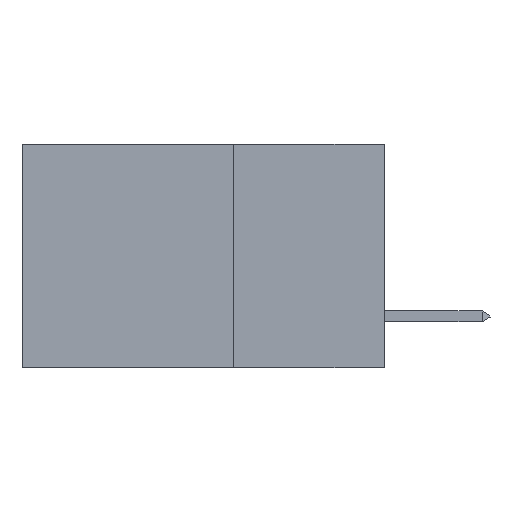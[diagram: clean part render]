
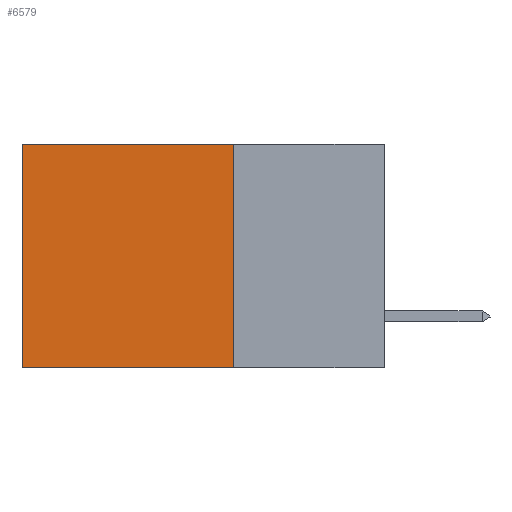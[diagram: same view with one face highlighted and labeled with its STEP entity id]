
A CAD part, left-side view. The second image highlights one B-rep face of the part: STEP entity #6579.
In plain terms, the highlighted planar face has unit normal (-1, 0, 0).
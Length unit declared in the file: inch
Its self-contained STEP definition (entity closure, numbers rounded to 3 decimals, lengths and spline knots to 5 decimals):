
#122 = EDGE_CURVE ( 'NONE', #7248, #6444, #5479, .T. ) ;
#138 = LINE ( 'NONE', #6933, #7232 ) ;
#564 = CARTESIAN_POINT ( 'NONE',  ( 0.2875, 0.25, -0.37 ) ) ;
#593 = CARTESIAN_POINT ( 'NONE',  ( 0.2875, 0.25, -0.37 ) ) ;
#656 = CARTESIAN_POINT ( 'NONE',  ( 0.2875, 0.25, 0. ) ) ;
#776 = ORIENTED_EDGE ( 'NONE', *, *, #122, .T. ) ;
#1270 = ORIENTED_EDGE ( 'NONE', *, *, #9127, .F. ) ;
#1490 = LINE ( 'NONE', #2116, #5525 ) ;
#1652 = CARTESIAN_POINT ( 'NONE',  ( 0.2875, 0.25, 0. ) ) ;
#2116 = CARTESIAN_POINT ( 'NONE',  ( 0.2875, 0.25, 0. ) ) ;
#2440 = VERTEX_POINT ( 'NONE', #564 ) ;
#2858 = DIRECTION ( 'NONE',  ( 0., 0., -1. ) ) ;
#2945 = EDGE_LOOP ( 'NONE', ( #3416, #3709, #1270, #776 ) ) ;
#3397 = VECTOR ( 'NONE', #7446, 39.37008 ) ;
#3416 = ORIENTED_EDGE ( 'NONE', *, *, #7971, .T. ) ;
#3709 = ORIENTED_EDGE ( 'NONE', *, *, #6536, .F. ) ;
#4109 = VECTOR ( 'NONE', #6903, 39.37008 ) ;
#4374 = CARTESIAN_POINT ( 'NONE',  ( 0.2875, 0.25, 0. ) ) ;
#4615 = DIRECTION ( 'NONE',  ( 0., 0., -1. ) ) ;
#4846 = LINE ( 'NONE', #593, #4109 ) ;
#5154 = CARTESIAN_POINT ( 'NONE',  ( 0.2875, 0.6, -0.37 ) ) ;
#5479 = LINE ( 'NONE', #4374, #3397 ) ;
#5525 = VECTOR ( 'NONE', #2858, 39.37008 ) ;
#5687 = AXIS2_PLACEMENT_3D ( 'NONE', #656, #6962, #4615 ) ;
#6236 = DIRECTION ( 'NONE',  ( 0., 0., -1. ) ) ;
#6444 = VERTEX_POINT ( 'NONE', #9734 ) ;
#6536 = EDGE_CURVE ( 'NONE', #2440, #8276, #4846, .T. ) ;
#6579 = ADVANCED_FACE ( 'NONE', ( #8725 ), #9194, .F. ) ;
#6903 = DIRECTION ( 'NONE',  ( 0., 1., 0. ) ) ;
#6933 = CARTESIAN_POINT ( 'NONE',  ( 0.2875, 0.6, 0. ) ) ;
#6962 = DIRECTION ( 'NONE',  ( 1., 0., 0. ) ) ;
#7232 = VECTOR ( 'NONE', #6236, 39.37008 ) ;
#7248 = VERTEX_POINT ( 'NONE', #1652 ) ;
#7446 = DIRECTION ( 'NONE',  ( 0., 1., 0. ) ) ;
#7971 = EDGE_CURVE ( 'NONE', #6444, #8276, #138, .T. ) ;
#8276 = VERTEX_POINT ( 'NONE', #5154 ) ;
#8725 = FACE_OUTER_BOUND ( 'NONE', #2945, .T. ) ;
#9127 = EDGE_CURVE ( 'NONE', #7248, #2440, #1490, .T. ) ;
#9194 = PLANE ( 'NONE',  #5687 ) ;
#9734 = CARTESIAN_POINT ( 'NONE',  ( 0.2875, 0.6, 0. ) ) ;
